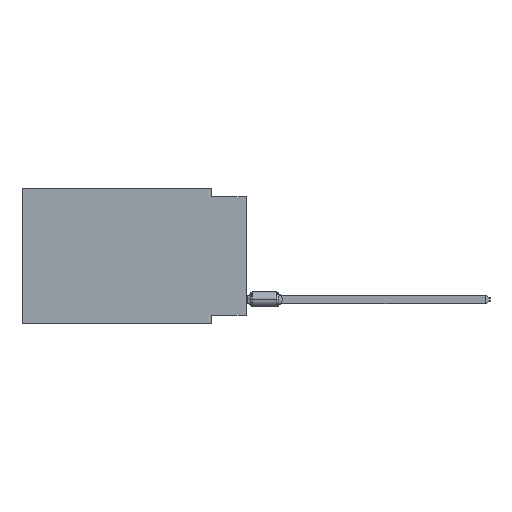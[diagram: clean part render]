
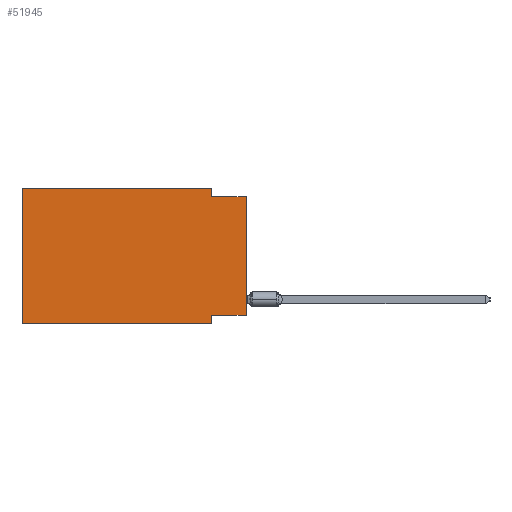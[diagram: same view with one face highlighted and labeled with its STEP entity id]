
A CAD part, left-side view. The second image highlights one B-rep face of the part: STEP entity #51945.
In plain terms, the highlighted planar face has unit normal (-1, 0, 0).
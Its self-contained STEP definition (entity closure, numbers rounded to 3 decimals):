
#771 = CARTESIAN_POINT ( 'NONE',  ( 0., 16.383, 0. ) ) ;
#1067 = LINE ( 'NONE', #77516, #11955 ) ;
#1977 = CARTESIAN_POINT ( 'NONE',  ( 0., 0., -0.635 ) ) ;
#2678 = VERTEX_POINT ( 'NONE', #21245 ) ;
#3440 = VECTOR ( 'NONE', #60895, 1000. ) ;
#4105 = CARTESIAN_POINT ( 'NONE',  ( 0., 16.383, -9.906 ) ) ;
#6056 = ORIENTED_EDGE ( 'NONE', *, *, #48834, .F. ) ;
#6851 = VECTOR ( 'NONE', #14860, 1000. ) ;
#9937 = CARTESIAN_POINT ( 'NONE',  ( 0., 16.383, 0. ) ) ;
#11955 = VECTOR ( 'NONE', #26155, 1000. ) ;
#12016 = CARTESIAN_POINT ( 'NONE',  ( 0., 2.54, 0. ) ) ;
#12992 = ORIENTED_EDGE ( 'NONE', *, *, #16508, .F. ) ;
#13047 = VERTEX_POINT ( 'NONE', #25572 ) ;
#14860 = DIRECTION ( 'NONE',  ( 0., 0., -1. ) ) ;
#16508 = EDGE_CURVE ( 'NONE', #77046, #75934, #67162, .T. ) ;
#17194 = EDGE_CURVE ( 'NONE', #43277, #61650, #52801, .T. ) ;
#18179 = EDGE_CURVE ( 'NONE', #2678, #38768, #23836, .T. ) ;
#21245 = CARTESIAN_POINT ( 'NONE',  ( 0., 2.54, -0.635 ) ) ;
#23836 = LINE ( 'NONE', #28867, #25035 ) ;
#25035 = VECTOR ( 'NONE', #28440, 1000. ) ;
#25572 = CARTESIAN_POINT ( 'NONE',  ( 0., 2.54, -9.906 ) ) ;
#26155 = DIRECTION ( 'NONE',  ( 0., 0., -1. ) ) ;
#26499 = CARTESIAN_POINT ( 'NONE',  ( 0., 0., -9.271 ) ) ;
#26844 = PLANE ( 'NONE',  #68056 ) ;
#27052 = ORIENTED_EDGE ( 'NONE', *, *, #18179, .F. ) ;
#27587 = DIRECTION ( 'NONE',  ( 0., 0., 1. ) ) ;
#28440 = DIRECTION ( 'NONE',  ( 0., -1., 0. ) ) ;
#28867 = CARTESIAN_POINT ( 'NONE',  ( 0., 0., -0.635 ) ) ;
#31121 = VECTOR ( 'NONE', #27587, 1000. ) ;
#32285 = CARTESIAN_POINT ( 'NONE',  ( 0., 16.383, 0. ) ) ;
#32471 = CARTESIAN_POINT ( 'NONE',  ( 0., 0., 0. ) ) ;
#32666 = ORIENTED_EDGE ( 'NONE', *, *, #41382, .T. ) ;
#37341 = EDGE_CURVE ( 'NONE', #43277, #38768, #37929, .T. ) ;
#37929 = LINE ( 'NONE', #32471, #40935 ) ;
#37948 = LINE ( 'NONE', #64246, #55398 ) ;
#38768 = VERTEX_POINT ( 'NONE', #1977 ) ;
#40211 = DIRECTION ( 'NONE',  ( 0., 0., -1. ) ) ;
#40935 = VECTOR ( 'NONE', #57953, 1000. ) ;
#41382 = EDGE_CURVE ( 'NONE', #75722, #13047, #37948, .T. ) ;
#43277 = VERTEX_POINT ( 'NONE', #66878 ) ;
#44877 = DIRECTION ( 'NONE',  ( 0., 1., 0. ) ) ;
#46599 = ORIENTED_EDGE ( 'NONE', *, *, #55363, .F. ) ;
#48064 = VECTOR ( 'NONE', #44877, 1000. ) ;
#48834 = EDGE_CURVE ( 'NONE', #75934, #2678, #1067, .T. ) ;
#50477 = DIRECTION ( 'NONE',  ( 0., -1., 0. ) ) ;
#51945 = ADVANCED_FACE ( 'NONE', ( #52745 ), #26844, .F. ) ;
#52745 = FACE_OUTER_BOUND ( 'NONE', #65574, .T. ) ;
#52801 = LINE ( 'NONE', #26499, #48064 ) ;
#54723 = ORIENTED_EDGE ( 'NONE', *, *, #37341, .T. ) ;
#55363 = EDGE_CURVE ( 'NONE', #75722, #77046, #72272, .T. ) ;
#55398 = VECTOR ( 'NONE', #50477, 1000. ) ;
#57953 = DIRECTION ( 'NONE',  ( 0., 0., 1. ) ) ;
#60895 = DIRECTION ( 'NONE',  ( 0., -1., 0. ) ) ;
#61650 = VERTEX_POINT ( 'NONE', #77463 ) ;
#63487 = ORIENTED_EDGE ( 'NONE', *, *, #17194, .F. ) ;
#64246 = CARTESIAN_POINT ( 'NONE',  ( 0., 16.383, -9.906 ) ) ;
#65574 = EDGE_LOOP ( 'NONE', ( #54723, #27052, #6056, #12992, #46599, #32666, #69261, #63487 ) ) ;
#66878 = CARTESIAN_POINT ( 'NONE',  ( 0., 0., -9.271 ) ) ;
#66933 = EDGE_CURVE ( 'NONE', #61650, #13047, #72079, .T. ) ;
#67162 = LINE ( 'NONE', #9937, #3440 ) ;
#68056 = AXIS2_PLACEMENT_3D ( 'NONE', #32285, #78630, #40211 ) ;
#69261 = ORIENTED_EDGE ( 'NONE', *, *, #66933, .F. ) ;
#71049 = CARTESIAN_POINT ( 'NONE',  ( 0., 16.383, 0. ) ) ;
#72079 = LINE ( 'NONE', #77521, #6851 ) ;
#72272 = LINE ( 'NONE', #71049, #31121 ) ;
#75722 = VERTEX_POINT ( 'NONE', #4105 ) ;
#75934 = VERTEX_POINT ( 'NONE', #12016 ) ;
#77046 = VERTEX_POINT ( 'NONE', #771 ) ;
#77463 = CARTESIAN_POINT ( 'NONE',  ( 0., 2.54, -9.271 ) ) ;
#77516 = CARTESIAN_POINT ( 'NONE',  ( 0., 2.54, 0. ) ) ;
#77521 = CARTESIAN_POINT ( 'NONE',  ( 0., 2.54, -9.906 ) ) ;
#78630 = DIRECTION ( 'NONE',  ( 1., 0., 0. ) ) ;
